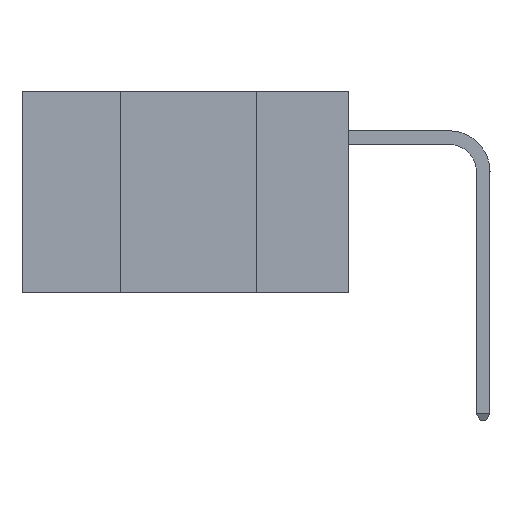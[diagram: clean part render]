
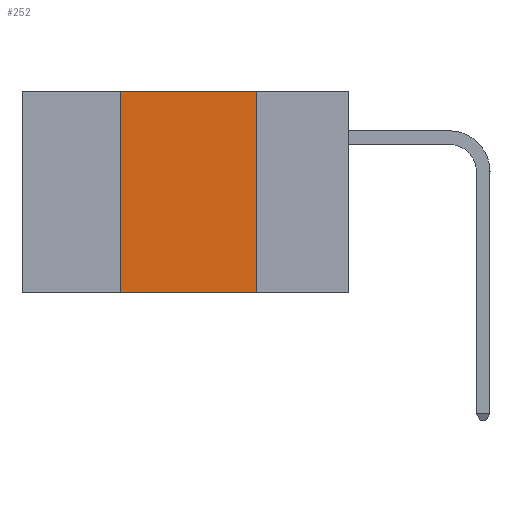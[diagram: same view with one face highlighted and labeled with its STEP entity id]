
A CAD part, left-side view. The second image highlights one B-rep face of the part: STEP entity #252.
In plain terms, the highlighted planar face has unit normal (-1, 0, 0).
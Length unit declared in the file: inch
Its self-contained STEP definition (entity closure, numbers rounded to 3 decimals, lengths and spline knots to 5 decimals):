
#252 = ADVANCED_FACE ( 'NONE', ( #18010 ), #25611, .F. ) ;
#402 = VECTOR ( 'NONE', #24960, 39.37008 ) ;
#620 = CARTESIAN_POINT ( 'NONE',  ( 0., 0.17, -0.37 ) ) ;
#1376 = EDGE_CURVE ( 'NONE', #8688, #40398, #17973, .T. ) ;
#1558 = VERTEX_POINT ( 'NONE', #3063 ) ;
#3063 = CARTESIAN_POINT ( 'NONE',  ( 0., 0.42, 0. ) ) ;
#5828 = DIRECTION ( 'NONE',  ( 0., 0., -1. ) ) ;
#8688 = VERTEX_POINT ( 'NONE', #49834 ) ;
#9750 = CARTESIAN_POINT ( 'NONE',  ( 0., 0.17, 0. ) ) ;
#9984 = ORIENTED_EDGE ( 'NONE', *, *, #41304, .T. ) ;
#10189 = VECTOR ( 'NONE', #33902, 39.37008 ) ;
#14032 = CARTESIAN_POINT ( 'NONE',  ( 0., 0.6, 0. ) ) ;
#14599 = DIRECTION ( 'NONE',  ( 0., -1., 0. ) ) ;
#16727 = VECTOR ( 'NONE', #5828, 39.37008 ) ;
#17265 = ORIENTED_EDGE ( 'NONE', *, *, #24320, .F. ) ;
#17957 = DIRECTION ( 'NONE',  ( 0., 0., -1. ) ) ;
#17973 = LINE ( 'NONE', #9750, #16727 ) ;
#18010 = FACE_OUTER_BOUND ( 'NONE', #37154, .T. ) ;
#20451 = VERTEX_POINT ( 'NONE', #44181 ) ;
#24099 = EDGE_CURVE ( 'NONE', #20451, #1558, #30302, .T. ) ;
#24320 = EDGE_CURVE ( 'NONE', #1558, #8688, #39912, .T. ) ;
#24960 = DIRECTION ( 'NONE',  ( 0., 0., 1. ) ) ;
#25611 = PLANE ( 'NONE',  #46552 ) ;
#28128 = LINE ( 'NONE', #37802, #38378 ) ;
#30010 = CARTESIAN_POINT ( 'NONE',  ( 0., 0.6, 0. ) ) ;
#30302 = LINE ( 'NONE', #36611, #402 ) ;
#33902 = DIRECTION ( 'NONE',  ( 0., -1., 0. ) ) ;
#36137 = ORIENTED_EDGE ( 'NONE', *, *, #24099, .F. ) ;
#36611 = CARTESIAN_POINT ( 'NONE',  ( 0., 0.42, 0. ) ) ;
#37154 = EDGE_LOOP ( 'NONE', ( #44474, #17265, #36137, #9984 ) ) ;
#37802 = CARTESIAN_POINT ( 'NONE',  ( 0., 0.6, -0.37 ) ) ;
#38378 = VECTOR ( 'NONE', #14599, 39.37008 ) ;
#39912 = LINE ( 'NONE', #30010, #10189 ) ;
#40398 = VERTEX_POINT ( 'NONE', #620 ) ;
#41096 = DIRECTION ( 'NONE',  ( 1., 0., 0. ) ) ;
#41304 = EDGE_CURVE ( 'NONE', #20451, #40398, #28128, .T. ) ;
#44181 = CARTESIAN_POINT ( 'NONE',  ( 0., 0.42, -0.37 ) ) ;
#44474 = ORIENTED_EDGE ( 'NONE', *, *, #1376, .F. ) ;
#46552 = AXIS2_PLACEMENT_3D ( 'NONE', #14032, #41096, #17957 ) ;
#49834 = CARTESIAN_POINT ( 'NONE',  ( 0., 0.17, 0. ) ) ;
